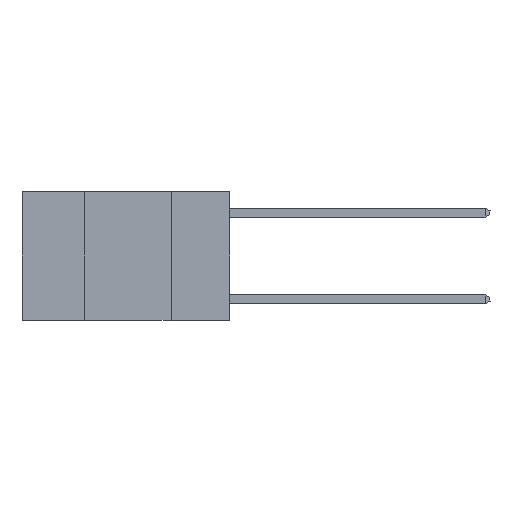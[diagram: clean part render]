
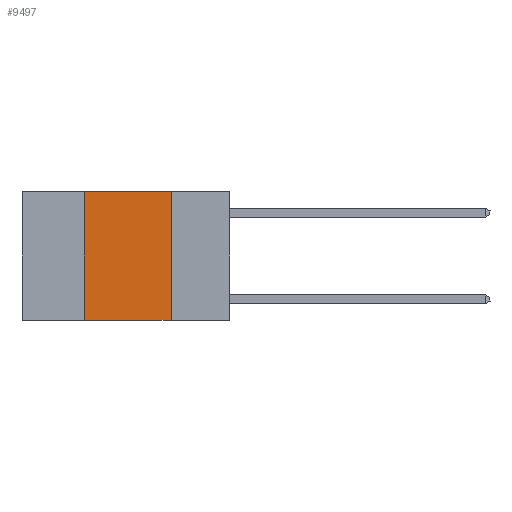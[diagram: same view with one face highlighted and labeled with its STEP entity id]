
A CAD part, left-side view. The second image highlights one B-rep face of the part: STEP entity #9497.
In plain terms, the highlighted planar face has unit normal (-1, 0, 0).
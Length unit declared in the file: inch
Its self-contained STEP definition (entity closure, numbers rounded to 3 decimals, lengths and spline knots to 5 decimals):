
#645 = VERTEX_POINT ( 'NONE', #13579 ) ;
#975 = DIRECTION ( 'NONE',  ( 0., 0., -1. ) ) ;
#1058 = CARTESIAN_POINT ( 'NONE',  ( 0., 0.17, 0. ) ) ;
#2704 = LINE ( 'NONE', #9410, #16350 ) ;
#4062 = DIRECTION ( 'NONE',  ( 0., 0., -1. ) ) ;
#4425 = DIRECTION ( 'NONE',  ( 0., -1., 0. ) ) ;
#4441 = DIRECTION ( 'NONE',  ( 0., -1., 0. ) ) ;
#4644 = CARTESIAN_POINT ( 'NONE',  ( 0., 0.6, -0.37 ) ) ;
#5889 = EDGE_CURVE ( 'NONE', #17431, #645, #16935, .T. ) ;
#6060 = DIRECTION ( 'NONE',  ( 0., 0., 1. ) ) ;
#6365 = AXIS2_PLACEMENT_3D ( 'NONE', #9270, #20592, #975 ) ;
#7185 = VERTEX_POINT ( 'NONE', #10084 ) ;
#7414 = ORIENTED_EDGE ( 'NONE', *, *, #18907, .F. ) ;
#7677 = LINE ( 'NONE', #4644, #20177 ) ;
#8665 = VECTOR ( 'NONE', #4062, 39.37008 ) ;
#9238 = CARTESIAN_POINT ( 'NONE',  ( 0., 0.17, -0.37 ) ) ;
#9270 = CARTESIAN_POINT ( 'NONE',  ( 0., 0.6, 0. ) ) ;
#9316 = EDGE_CURVE ( 'NONE', #645, #7185, #2704, .T. ) ;
#9410 = CARTESIAN_POINT ( 'NONE',  ( 0., 0.6, 0. ) ) ;
#9497 = ADVANCED_FACE ( 'NONE', ( #17548 ), #17442, .F. ) ;
#9854 = VERTEX_POINT ( 'NONE', #9238 ) ;
#10084 = CARTESIAN_POINT ( 'NONE',  ( 0., 0.17, 0. ) ) ;
#10856 = EDGE_CURVE ( 'NONE', #17431, #9854, #7677, .T. ) ;
#11134 = ORIENTED_EDGE ( 'NONE', *, *, #10856, .T. ) ;
#11170 = EDGE_LOOP ( 'NONE', ( #7414, #12847, #17325, #11134 ) ) ;
#12847 = ORIENTED_EDGE ( 'NONE', *, *, #9316, .F. ) ;
#12985 = CARTESIAN_POINT ( 'NONE',  ( 0., 0.42, -0.37 ) ) ;
#13579 = CARTESIAN_POINT ( 'NONE',  ( 0., 0.42, 0. ) ) ;
#13589 = VECTOR ( 'NONE', #6060, 39.37008 ) ;
#16350 = VECTOR ( 'NONE', #4441, 39.37008 ) ;
#16935 = LINE ( 'NONE', #20398, #13589 ) ;
#17325 = ORIENTED_EDGE ( 'NONE', *, *, #5889, .F. ) ;
#17431 = VERTEX_POINT ( 'NONE', #12985 ) ;
#17442 = PLANE ( 'NONE',  #6365 ) ;
#17548 = FACE_OUTER_BOUND ( 'NONE', #11170, .T. ) ;
#18615 = LINE ( 'NONE', #1058, #8665 ) ;
#18907 = EDGE_CURVE ( 'NONE', #7185, #9854, #18615, .T. ) ;
#20177 = VECTOR ( 'NONE', #4425, 39.37008 ) ;
#20398 = CARTESIAN_POINT ( 'NONE',  ( 0., 0.42, 0. ) ) ;
#20592 = DIRECTION ( 'NONE',  ( 1., 0., 0. ) ) ;
